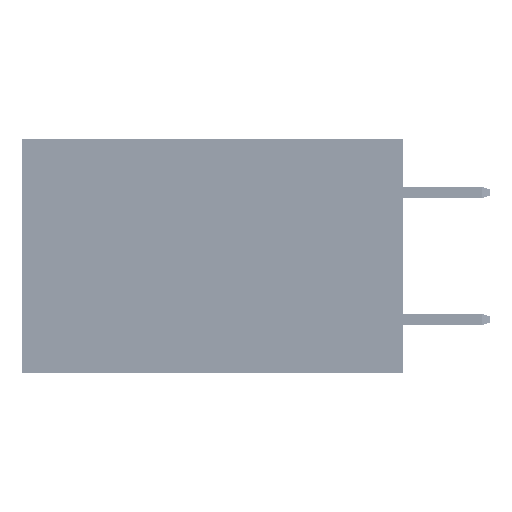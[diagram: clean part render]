
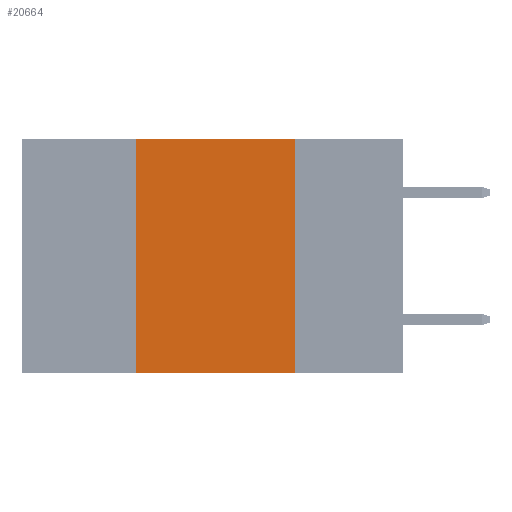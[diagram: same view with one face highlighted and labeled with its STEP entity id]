
A CAD part, left-side view. The second image highlights one B-rep face of the part: STEP entity #20664.
In plain terms, the highlighted planar face has unit normal (-1, 0, 0).
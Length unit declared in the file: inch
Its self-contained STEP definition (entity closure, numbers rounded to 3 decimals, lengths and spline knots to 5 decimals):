
#467 = VECTOR ( 'NONE', #22762, 39.37008 ) ;
#865 = VERTEX_POINT ( 'NONE', #15158 ) ;
#1026 = ORIENTED_EDGE ( 'NONE', *, *, #37999, .F. ) ;
#1419 = VERTEX_POINT ( 'NONE', #47455 ) ;
#3174 = CARTESIAN_POINT ( 'NONE',  ( 0., 0.42, 0. ) ) ;
#3499 = EDGE_CURVE ( 'NONE', #12269, #47760, #17927, .T. ) ;
#4561 = DIRECTION ( 'NONE',  ( 0., 0., -1. ) ) ;
#5753 = DIRECTION ( 'NONE',  ( 0., 0., -1. ) ) ;
#7255 = LINE ( 'NONE', #45815, #467 ) ;
#7513 = CARTESIAN_POINT ( 'NONE',  ( 0., 0.6, -0.37 ) ) ;
#8383 = ORIENTED_EDGE ( 'NONE', *, *, #21609, .T. ) ;
#11548 = VECTOR ( 'NONE', #27051, 39.37008 ) ;
#12269 = VERTEX_POINT ( 'NONE', #48118 ) ;
#13497 = VECTOR ( 'NONE', #5753, 39.37008 ) ;
#15158 = CARTESIAN_POINT ( 'NONE',  ( 0., 0.17, -0.37 ) ) ;
#16843 = ORIENTED_EDGE ( 'NONE', *, *, #28027, .F. ) ;
#17927 = LINE ( 'NONE', #3174, #39238 ) ;
#20664 = ADVANCED_FACE ( 'NONE', ( #23381 ), #38831, .F. ) ;
#21609 = EDGE_CURVE ( 'NONE', #12269, #865, #23257, .T. ) ;
#22762 = DIRECTION ( 'NONE',  ( 0., -1., 0. ) ) ;
#23257 = LINE ( 'NONE', #7513, #11548 ) ;
#23381 = FACE_OUTER_BOUND ( 'NONE', #29752, .T. ) ;
#24612 = CARTESIAN_POINT ( 'NONE',  ( 0., 0.42, 0. ) ) ;
#26883 = AXIS2_PLACEMENT_3D ( 'NONE', #27170, #39087, #4561 ) ;
#27051 = DIRECTION ( 'NONE',  ( 0., -1., 0. ) ) ;
#27170 = CARTESIAN_POINT ( 'NONE',  ( 0., 0.6, 0. ) ) ;
#28027 = EDGE_CURVE ( 'NONE', #1419, #865, #40778, .T. ) ;
#29752 = EDGE_LOOP ( 'NONE', ( #16843, #1026, #34442, #8383 ) ) ;
#34442 = ORIENTED_EDGE ( 'NONE', *, *, #3499, .F. ) ;
#37999 = EDGE_CURVE ( 'NONE', #47760, #1419, #7255, .T. ) ;
#38831 = PLANE ( 'NONE',  #26883 ) ;
#39087 = DIRECTION ( 'NONE',  ( 1., 0., 0. ) ) ;
#39238 = VECTOR ( 'NONE', #49598, 39.37008 ) ;
#40526 = CARTESIAN_POINT ( 'NONE',  ( 0., 0.17, 0. ) ) ;
#40778 = LINE ( 'NONE', #40526, #13497 ) ;
#45815 = CARTESIAN_POINT ( 'NONE',  ( 0., 0.6, 0. ) ) ;
#47455 = CARTESIAN_POINT ( 'NONE',  ( 0., 0.17, 0. ) ) ;
#47760 = VERTEX_POINT ( 'NONE', #24612 ) ;
#48118 = CARTESIAN_POINT ( 'NONE',  ( 0., 0.42, -0.37 ) ) ;
#49598 = DIRECTION ( 'NONE',  ( 0., 0., 1. ) ) ;
